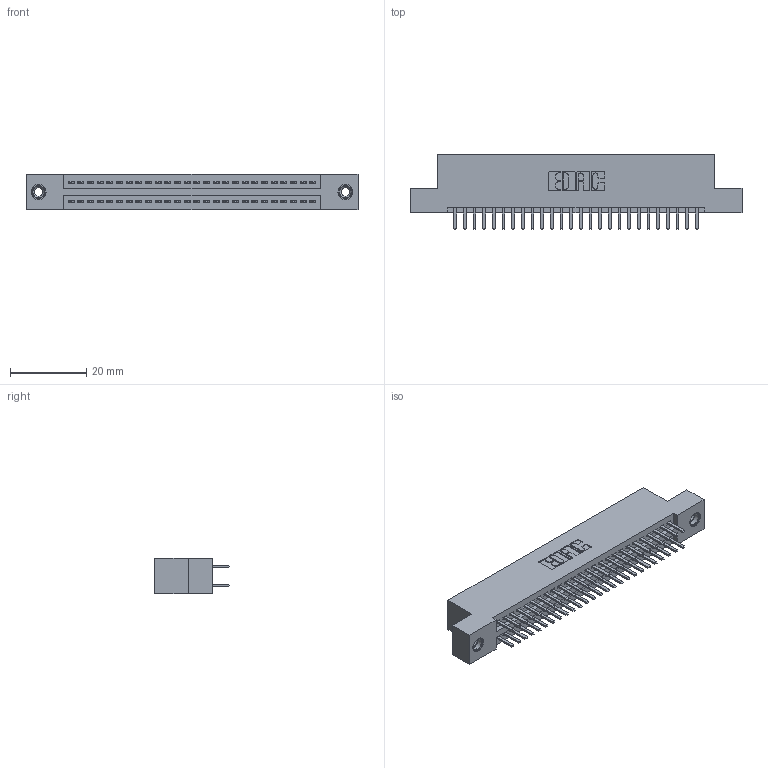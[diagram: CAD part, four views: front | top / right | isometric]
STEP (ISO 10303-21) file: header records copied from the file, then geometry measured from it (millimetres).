
FILE_DESCRIPTION (( 'STEP AP203' ), '1' );
FILE_NAME ('395-052-520-208.STEP', '2018-11-20T20:38:57', ( '' ), ( '' ), 'SwSTEP 2.0', 'SolidWorks 2016', '' );
FILE_SCHEMA (( 'CONFIG_CONTROL_DESIGN' ));
Length unit declared in the file: inch
Products named in the file (4): 345 Part_Flush Mounting Lugs - 0.156 Dia-TI; 345-292-001_345-293-120; 395-052-520-208; 345-250-001_345-250-003-102
Assembly tree (55 placements, depth 2):
  395-052-520-208
    345 Part_Flush Mounting Lugs - 0.156 Dia-TI
    345-292-001_345-293-120  x52
    345-250-001_345-250-003-102  x2
Bounding box: 87.25 x 19.68 x 9.4 mm (x, y, z)
Volume: 8297.6 mm3; surface area: 11920.1 mm2
Topology: 55 solids, 55 shells, 2994 faces, 8641 edges, 5614 vertices
Faces by surface type: plane 1932, cylinder 1046, cone 12, torus 4
Entity records: 23854 total; most frequent: CARTESIAN_POINT 4007, ORIENTED_EDGE 3922, DIRECTION 3567, EDGE_CURVE 1961, LINE 1701, VECTOR 1701, VERTEX_POINT 1300, AXIS2_PLACEMENT_3D 933
